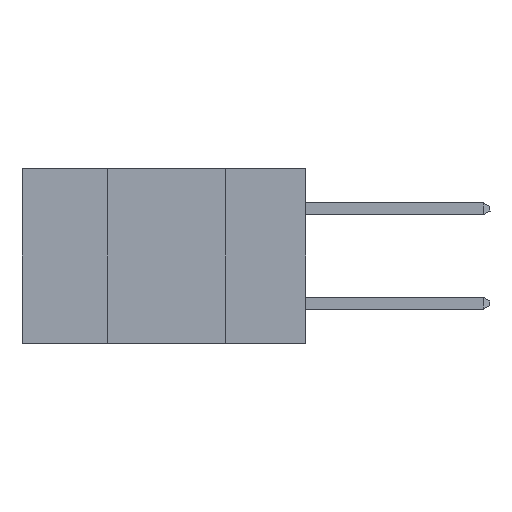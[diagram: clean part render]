
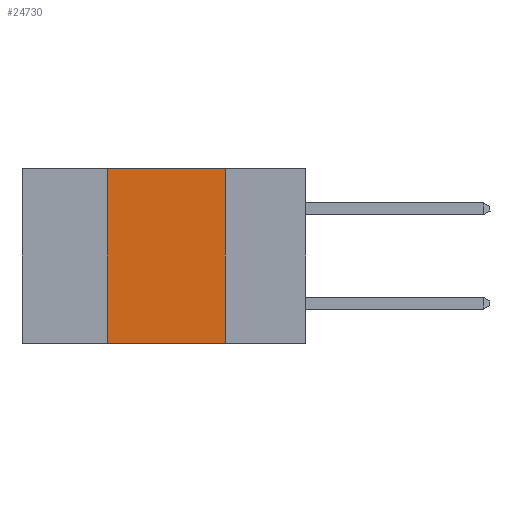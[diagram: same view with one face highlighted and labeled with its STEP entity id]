
A CAD part, left-side view. The second image highlights one B-rep face of the part: STEP entity #24730.
In plain terms, the highlighted planar face has unit normal (-1, 0, 0).
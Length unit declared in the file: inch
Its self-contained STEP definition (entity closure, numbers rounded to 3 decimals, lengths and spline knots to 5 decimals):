
#2336 = LINE ( 'NONE', #16102, #16851 ) ;
#2604 = VECTOR ( 'NONE', #11915, 39.37008 ) ;
#2675 = CARTESIAN_POINT ( 'NONE',  ( 0., 0.6, -0.37 ) ) ;
#3988 = ORIENTED_EDGE ( 'NONE', *, *, #21326, .F. ) ;
#5586 = ORIENTED_EDGE ( 'NONE', *, *, #6273, .T. ) ;
#6273 = EDGE_CURVE ( 'NONE', #18155, #12528, #25161, .T. ) ;
#6453 = DIRECTION ( 'NONE',  ( 0., -1., 0. ) ) ;
#6542 = CARTESIAN_POINT ( 'NONE',  ( 0., 0.17, -0.37 ) ) ;
#7658 = CARTESIAN_POINT ( 'NONE',  ( 0., 0.17, 0. ) ) ;
#8653 = EDGE_LOOP ( 'NONE', ( #3988, #18250, #9649, #5586 ) ) ;
#8741 = DIRECTION ( 'NONE',  ( 1., 0., 0. ) ) ;
#9649 = ORIENTED_EDGE ( 'NONE', *, *, #21903, .F. ) ;
#10999 = VERTEX_POINT ( 'NONE', #24322 ) ;
#11051 = CARTESIAN_POINT ( 'NONE',  ( 0., 0.6, 0. ) ) ;
#11915 = DIRECTION ( 'NONE',  ( 0., 0., -1. ) ) ;
#12209 = LINE ( 'NONE', #12270, #2604 ) ;
#12246 = AXIS2_PLACEMENT_3D ( 'NONE', #18995, #8741, #14847 ) ;
#12270 = CARTESIAN_POINT ( 'NONE',  ( 0., 0.17, 0. ) ) ;
#12528 = VERTEX_POINT ( 'NONE', #6542 ) ;
#14250 = VECTOR ( 'NONE', #19613, 39.37008 ) ;
#14847 = DIRECTION ( 'NONE',  ( 0., 0., -1. ) ) ;
#15924 = LINE ( 'NONE', #11051, #16223 ) ;
#16102 = CARTESIAN_POINT ( 'NONE',  ( 0., 0.42, 0. ) ) ;
#16223 = VECTOR ( 'NONE', #6453, 39.37008 ) ;
#16851 = VECTOR ( 'NONE', #24621, 39.37008 ) ;
#16955 = PLANE ( 'NONE',  #12246 ) ;
#18155 = VERTEX_POINT ( 'NONE', #24606 ) ;
#18250 = ORIENTED_EDGE ( 'NONE', *, *, #21622, .F. ) ;
#18995 = CARTESIAN_POINT ( 'NONE',  ( 0., 0.6, 0. ) ) ;
#19613 = DIRECTION ( 'NONE',  ( 0., -1., 0. ) ) ;
#21056 = FACE_OUTER_BOUND ( 'NONE', #8653, .T. ) ;
#21326 = EDGE_CURVE ( 'NONE', #25366, #12528, #12209, .T. ) ;
#21622 = EDGE_CURVE ( 'NONE', #10999, #25366, #15924, .T. ) ;
#21903 = EDGE_CURVE ( 'NONE', #18155, #10999, #2336, .T. ) ;
#24322 = CARTESIAN_POINT ( 'NONE',  ( 0., 0.42, 0. ) ) ;
#24606 = CARTESIAN_POINT ( 'NONE',  ( 0., 0.42, -0.37 ) ) ;
#24621 = DIRECTION ( 'NONE',  ( 0., 0., 1. ) ) ;
#24730 = ADVANCED_FACE ( 'NONE', ( #21056 ), #16955, .F. ) ;
#25161 = LINE ( 'NONE', #2675, #14250 ) ;
#25366 = VERTEX_POINT ( 'NONE', #7658 ) ;
